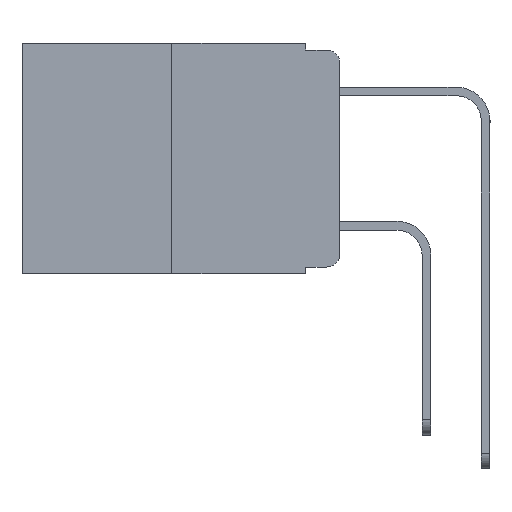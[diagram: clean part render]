
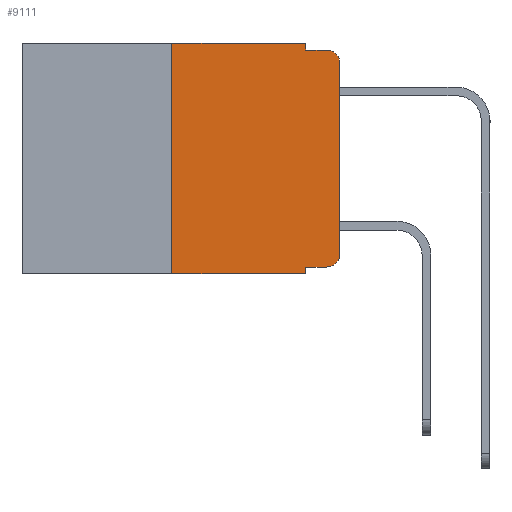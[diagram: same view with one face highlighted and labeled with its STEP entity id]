
A CAD part, left-side view. The second image highlights one B-rep face of the part: STEP entity #9111.
In plain terms, the highlighted planar face has unit normal (-1, 0, 0).
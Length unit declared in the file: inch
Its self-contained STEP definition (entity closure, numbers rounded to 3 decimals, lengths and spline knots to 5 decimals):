
#38 = VECTOR ( 'NONE', #3601, 39.37008 ) ;
#105 = VERTEX_POINT ( 'NONE', #6031 ) ;
#168 = CARTESIAN_POINT ( 'NONE',  ( 0., 0.051, 0. ) ) ;
#733 = ORIENTED_EDGE ( 'NONE', *, *, #8715, .T. ) ;
#950 = EDGE_LOOP ( 'NONE', ( #2072, #733, #5670, #7593, #1076, #1396, #8940, #7739, #10463, #7895 ) ) ;
#1076 = ORIENTED_EDGE ( 'NONE', *, *, #1232, .F. ) ;
#1198 = LINE ( 'NONE', #168, #6647 ) ;
#1232 = EDGE_CURVE ( 'NONE', #11604, #105, #10654, .T. ) ;
#1396 = ORIENTED_EDGE ( 'NONE', *, *, #5477, .F. ) ;
#1398 = VERTEX_POINT ( 'NONE', #5707 ) ;
#1715 = DIRECTION ( 'NONE',  ( 0., 0., -1. ) ) ;
#1894 = LINE ( 'NONE', #7008, #6999 ) ;
#1909 = DIRECTION ( 'NONE',  ( -1., 0., 0. ) ) ;
#2072 = ORIENTED_EDGE ( 'NONE', *, *, #9335, .T. ) ;
#2369 = VECTOR ( 'NONE', #5924, 39.37008 ) ;
#2772 = CARTESIAN_POINT ( 'NONE',  ( 0., 0.051, -0.01 ) ) ;
#3331 = VERTEX_POINT ( 'NONE', #6638 ) ;
#3563 = VECTOR ( 'NONE', #10769, 39.37008 ) ;
#3601 = DIRECTION ( 'NONE',  ( 0., 0., 1. ) ) ;
#3780 = DIRECTION ( 'NONE',  ( 1., 0., 0. ) ) ;
#3811 = DIRECTION ( 'NONE',  ( 0., -1., 0. ) ) ;
#3916 = VECTOR ( 'NONE', #8633, 39.37008 ) ;
#4013 = DIRECTION ( 'NONE',  ( -1., 0., 0. ) ) ;
#4357 = VERTEX_POINT ( 'NONE', #8638 ) ;
#4702 = EDGE_CURVE ( 'NONE', #4357, #5611, #12528, .T. ) ;
#4753 = PLANE ( 'NONE',  #4798 ) ;
#4798 = AXIS2_PLACEMENT_3D ( 'NONE', #7732, #3780, #10487 ) ;
#5252 = LINE ( 'NONE', #6755, #38 ) ;
#5280 = CARTESIAN_POINT ( 'NONE',  ( 0., 0.25, 0. ) ) ;
#5477 = EDGE_CURVE ( 'NONE', #4357, #11604, #5252, .T. ) ;
#5611 = VERTEX_POINT ( 'NONE', #7910 ) ;
#5670 = ORIENTED_EDGE ( 'NONE', *, *, #6799, .F. ) ;
#5707 = CARTESIAN_POINT ( 'NONE',  ( 0., 0.02, -0.01 ) ) ;
#5820 = CARTESIAN_POINT ( 'NONE',  ( 0., 0.051, 0. ) ) ;
#5924 = DIRECTION ( 'NONE',  ( 0., -1., 0. ) ) ;
#6031 = CARTESIAN_POINT ( 'NONE',  ( 0., 0.051, 0. ) ) ;
#6106 = FACE_OUTER_BOUND ( 'NONE', #950, .T. ) ;
#6123 = CARTESIAN_POINT ( 'NONE',  ( 0., 0., 0. ) ) ;
#6136 = EDGE_CURVE ( 'NONE', #105, #10227, #10293, .T. ) ;
#6255 = LINE ( 'NONE', #6123, #3563 ) ;
#6638 = CARTESIAN_POINT ( 'NONE',  ( 0., 0.051, -0.333 ) ) ;
#6647 = VECTOR ( 'NONE', #7342, 39.37008 ) ;
#6755 = CARTESIAN_POINT ( 'NONE',  ( 0., 0.25, 0. ) ) ;
#6799 = EDGE_CURVE ( 'NONE', #10227, #1398, #11237, .T. ) ;
#6999 = VECTOR ( 'NONE', #12507, 39.37008 ) ;
#7008 = CARTESIAN_POINT ( 'NONE',  ( 0., 0.051, -0.333 ) ) ;
#7342 = DIRECTION ( 'NONE',  ( 0., 0., -1. ) ) ;
#7447 = CARTESIAN_POINT ( 'NONE',  ( 0., 0., -0.313 ) ) ;
#7593 = ORIENTED_EDGE ( 'NONE', *, *, #6136, .F. ) ;
#7732 = CARTESIAN_POINT ( 'NONE',  ( 0., 0.473, 0. ) ) ;
#7739 = ORIENTED_EDGE ( 'NONE', *, *, #11631, .F. ) ;
#7838 = VECTOR ( 'NONE', #1715, 39.37008 ) ;
#7895 = ORIENTED_EDGE ( 'NONE', *, *, #10510, .T. ) ;
#7910 = CARTESIAN_POINT ( 'NONE',  ( 0., 0.051, -0.343 ) ) ;
#7946 = CARTESIAN_POINT ( 'NONE',  ( 0., 0.02, -0.03 ) ) ;
#8072 = CIRCLE ( 'NONE', #10992, 0.02 ) ;
#8363 = CARTESIAN_POINT ( 'NONE',  ( 0., 0.473, 0. ) ) ;
#8589 = CARTESIAN_POINT ( 'NONE',  ( 0., 0.02, -0.333 ) ) ;
#8633 = DIRECTION ( 'NONE',  ( 0., -1., 0. ) ) ;
#8638 = CARTESIAN_POINT ( 'NONE',  ( 0., 0.25, -0.343 ) ) ;
#8683 = VERTEX_POINT ( 'NONE', #11474 ) ;
#8715 = EDGE_CURVE ( 'NONE', #8683, #1398, #8072, .T. ) ;
#8849 = VECTOR ( 'NONE', #3811, 39.37008 ) ;
#8911 = DIRECTION ( 'NONE',  ( 0., 0., -1. ) ) ;
#8926 = CIRCLE ( 'NONE', #9429, 0.02 ) ;
#8940 = ORIENTED_EDGE ( 'NONE', *, *, #4702, .T. ) ;
#9111 = ADVANCED_FACE ( 'NONE', ( #6106 ), #4753, .F. ) ;
#9335 = EDGE_CURVE ( 'NONE', #10806, #8683, #6255, .T. ) ;
#9429 = AXIS2_PLACEMENT_3D ( 'NONE', #9815, #4013, #10703 ) ;
#9815 = CARTESIAN_POINT ( 'NONE',  ( 0., 0.02, -0.313 ) ) ;
#9929 = EDGE_CURVE ( 'NONE', #3331, #11349, #1894, .T. ) ;
#9952 = CARTESIAN_POINT ( 'NONE',  ( 0., 0.473, -0.343 ) ) ;
#10227 = VERTEX_POINT ( 'NONE', #11965 ) ;
#10293 = LINE ( 'NONE', #5820, #7838 ) ;
#10463 = ORIENTED_EDGE ( 'NONE', *, *, #9929, .T. ) ;
#10487 = DIRECTION ( 'NONE',  ( 0., 0., -1. ) ) ;
#10510 = EDGE_CURVE ( 'NONE', #11349, #10806, #8926, .T. ) ;
#10654 = LINE ( 'NONE', #8363, #3916 ) ;
#10703 = DIRECTION ( 'NONE',  ( 0., 0., -1. ) ) ;
#10769 = DIRECTION ( 'NONE',  ( 0., 0., 1. ) ) ;
#10806 = VERTEX_POINT ( 'NONE', #7447 ) ;
#10992 = AXIS2_PLACEMENT_3D ( 'NONE', #7946, #1909, #8911 ) ;
#11237 = LINE ( 'NONE', #2772, #8849 ) ;
#11349 = VERTEX_POINT ( 'NONE', #8589 ) ;
#11474 = CARTESIAN_POINT ( 'NONE',  ( 0., 0., -0.03 ) ) ;
#11604 = VERTEX_POINT ( 'NONE', #5280 ) ;
#11631 = EDGE_CURVE ( 'NONE', #3331, #5611, #1198, .T. ) ;
#11965 = CARTESIAN_POINT ( 'NONE',  ( 0., 0.051, -0.01 ) ) ;
#12507 = DIRECTION ( 'NONE',  ( 0., -1., 0. ) ) ;
#12528 = LINE ( 'NONE', #9952, #2369 ) ;
